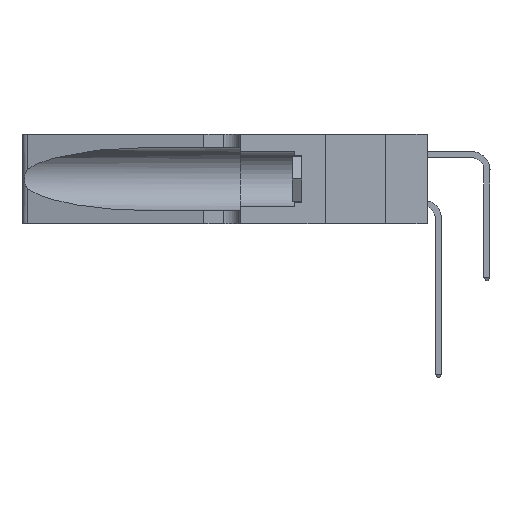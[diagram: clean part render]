
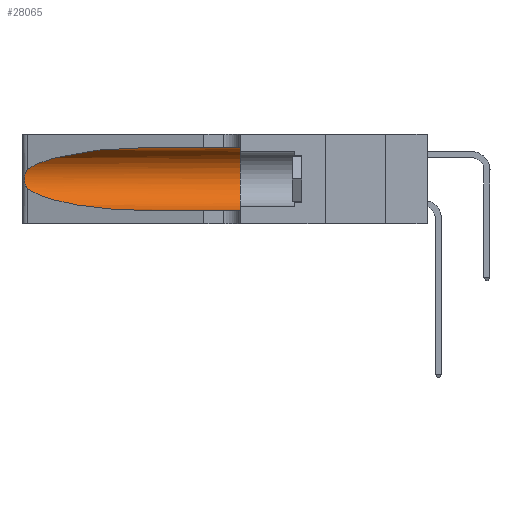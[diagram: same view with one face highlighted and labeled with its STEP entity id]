
A CAD part, left-side view. The second image highlights one B-rep face of the part: STEP entity #28065.
In plain terms, the highlighted cylindrical face has radius 3.308 mm (diameter 6.617 mm), a partial arc.
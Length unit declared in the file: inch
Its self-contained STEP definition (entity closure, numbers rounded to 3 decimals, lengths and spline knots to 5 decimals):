
#1088 = VERTEX_POINT ( 'NONE', #12390 ) ;
#1536 = AXIS2_PLACEMENT_3D ( 'NONE', #12603, #27786, #14799 ) ;
#1620 = CARTESIAN_POINT ( 'NONE',  ( 0.25856, 1.23593, 0.16098 ) ) ;
#2555 = EDGE_CURVE ( 'NONE', #1088, #3477, #3998, .T. ) ;
#2983 = DIRECTION ( 'NONE',  ( 0., -1., 0. ) ) ;
#3477 = VERTEX_POINT ( 'NONE', #13409 ) ;
#3913 = CARTESIAN_POINT ( 'NONE',  ( 0.25487, 1.22718, 0.14631 ) ) ;
#3923 = CARTESIAN_POINT ( 'NONE',  ( 0.25639, 1.23186, 0.15144 ) ) ;
#3998 = B_SPLINE_CURVE_WITH_KNOTS ( 'NONE', 3,
 ( #19181, #21332, #8282, #23526, #10497, #25715, #12701, #27890, #14899, #1620, #17091, #3923, #19275, #6166 ),
 .UNSPECIFIED., .F., .F.,
 ( 4, 2, 2, 2, 2, 2, 4 ),
 ( 0., 0.00027, 0.00053, 0.00107, 0.0016, 0.00187, 0.00214 ),
 .UNSPECIFIED. ) ;
#5432 = VECTOR ( 'NONE', #28395, 39.37008 ) ;
#5840 = CARTESIAN_POINT ( 'NONE',  ( 0.1305, 0.35, 0.31525 ) ) ;
#6016 = VERTEX_POINT ( 'NONE', #20432 ) ;
#6166 = CARTESIAN_POINT ( 'NONE',  ( 0.25487, 1.22718, 0.14631 ) ) ;
#6341 = FACE_OUTER_BOUND ( 'NONE', #9222, .T. ) ;
#6517 = DIRECTION ( 'NONE',  ( 0., 0., -1. ) ) ;
#6996 = DIRECTION ( 'NONE',  ( 0., -1., 0. ) ) ;
#8065 = CIRCLE ( 'NONE', #1536, 0.13025 ) ;
#8282 = CARTESIAN_POINT ( 'NONE',  ( 0.25639, 1.23184, 0.21858 ) ) ;
#8372 = CARTESIAN_POINT ( 'NONE',  ( 0.1305, 0.72297, 0.05475 ) ) ;
#9222 = EDGE_LOOP ( 'NONE', ( #16063, #11621, #13001, #24546, #14367, #15057 ) ) ;
#9246 = VERTEX_POINT ( 'NONE', #5840 ) ;
#9390 = VERTEX_POINT ( 'NONE', #28125 ) ;
#9672 =( BOUNDED_CURVE ( )  B_SPLINE_CURVE ( 3, ( #18338, #26934, #24857, #11829 ),
 .UNSPECIFIED., .F., .T. ) 
 B_SPLINE_CURVE_WITH_KNOTS ( ( 4, 4 ),
 ( 1.5708, 2.84003 ),
 .UNSPECIFIED. ) 
 CURVE ( )  GEOMETRIC_REPRESENTATION_ITEM ( )  RATIONAL_B_SPLINE_CURVE ( ( 1., 0.87, 0.87, 1. ) ) 
 REPRESENTATION_ITEM ( '' )  );
#10497 = CARTESIAN_POINT ( 'NONE',  ( 0.25854, 1.2359, 0.20912 ) ) ;
#11621 = ORIENTED_EDGE ( 'NONE', *, *, #2555, .T. ) ;
#11829 = CARTESIAN_POINT ( 'NONE',  ( 0.25487, 1.22718, 0.22369 ) ) ;
#12390 = CARTESIAN_POINT ( 'NONE',  ( 0.25487, 1.22718, 0.22369 ) ) ;
#12603 = CARTESIAN_POINT ( 'NONE',  ( 0.1305, 0.35, 0.185 ) ) ;
#12701 = CARTESIAN_POINT ( 'NONE',  ( 0.26075, 1.23896, 0.19203 ) ) ;
#13001 = ORIENTED_EDGE ( 'NONE', *, *, #20253, .T. ) ;
#13203 = CARTESIAN_POINT ( 'NONE',  ( 0.1305, 1.61858, 0.05475 ) ) ;
#13409 = CARTESIAN_POINT ( 'NONE',  ( 0.25487, 1.22718, 0.14631 ) ) ;
#14367 = ORIENTED_EDGE ( 'NONE', *, *, #20207, .F. ) ;
#14752 =( BOUNDED_CURVE ( )  B_SPLINE_CURVE ( 3, ( #3913, #17085, #21414, #8372 ),
 .UNSPECIFIED., .F., .T. ) 
 B_SPLINE_CURVE_WITH_KNOTS ( ( 4, 4 ),
 ( 3.44316, 4.71239 ),
 .UNSPECIFIED. ) 
 CURVE ( )  GEOMETRIC_REPRESENTATION_ITEM ( )  RATIONAL_B_SPLINE_CURVE ( ( 1., 0.87, 0.87, 1. ) ) 
 REPRESENTATION_ITEM ( '' )  );
#14799 = DIRECTION ( 'NONE',  ( 0., 0., 1. ) ) ;
#14899 = CARTESIAN_POINT ( 'NONE',  ( 0.26017, 1.23833, 0.17102 ) ) ;
#15057 = ORIENTED_EDGE ( 'NONE', *, *, #26070, .F. ) ;
#16063 = ORIENTED_EDGE ( 'NONE', *, *, #21930, .T. ) ;
#17021 = VECTOR ( 'NONE', #2983, 39.37008 ) ;
#17085 = CARTESIAN_POINT ( 'NONE',  ( 0.2373, 1.15595, 0.08982 ) ) ;
#17091 = CARTESIAN_POINT ( 'NONE',  ( 0.25789, 1.23486, 0.15765 ) ) ;
#18338 = CARTESIAN_POINT ( 'NONE',  ( 0.1305, 0.72297, 0.31525 ) ) ;
#18398 = CARTESIAN_POINT ( 'NONE',  ( 0.1305, 1.61858, 0.31525 ) ) ;
#19181 = CARTESIAN_POINT ( 'NONE',  ( 0.25487, 1.22718, 0.22369 ) ) ;
#19275 = CARTESIAN_POINT ( 'NONE',  ( 0.25555, 1.22993, 0.14849 ) ) ;
#20082 = CARTESIAN_POINT ( 'NONE',  ( 0.1305, 1.61858, 0.185 ) ) ;
#20207 = EDGE_CURVE ( 'NONE', #9246, #6016, #8065, .T. ) ;
#20253 = EDGE_CURVE ( 'NONE', #3477, #9390, #14752, .T. ) ;
#20432 = CARTESIAN_POINT ( 'NONE',  ( 0.1305, 0.35, 0.05475 ) ) ;
#20837 = AXIS2_PLACEMENT_3D ( 'NONE', #20082, #6996, #6517 ) ;
#21332 = CARTESIAN_POINT ( 'NONE',  ( 0.25555, 1.22994, 0.2215 ) ) ;
#21414 = CARTESIAN_POINT ( 'NONE',  ( 0.18966, 0.96281, 0.05475 ) ) ;
#21930 = EDGE_CURVE ( 'NONE', #27591, #1088, #9672, .T. ) ;
#22356 = CYLINDRICAL_SURFACE ( 'NONE', #20837, 0.13025 ) ;
#22808 = LINE ( 'NONE', #13203, #5432 ) ;
#23526 = CARTESIAN_POINT ( 'NONE',  ( 0.25787, 1.23484, 0.2124 ) ) ;
#24546 = ORIENTED_EDGE ( 'NONE', *, *, #25156, .T. ) ;
#24857 = CARTESIAN_POINT ( 'NONE',  ( 0.2373, 1.15595, 0.28018 ) ) ;
#25156 = EDGE_CURVE ( 'NONE', #9390, #6016, #22808, .T. ) ;
#25715 = CARTESIAN_POINT ( 'NONE',  ( 0.26018, 1.23835, 0.19895 ) ) ;
#26070 = EDGE_CURVE ( 'NONE', #27591, #9246, #27865, .T. ) ;
#26934 = CARTESIAN_POINT ( 'NONE',  ( 0.18966, 0.96281, 0.31525 ) ) ;
#27591 = VERTEX_POINT ( 'NONE', #28076 ) ;
#27786 = DIRECTION ( 'NONE',  ( 0., 1., 0. ) ) ;
#27865 = LINE ( 'NONE', #18398, #17021 ) ;
#27890 = CARTESIAN_POINT ( 'NONE',  ( 0.26075, 1.23896, 0.178 ) ) ;
#28065 = ADVANCED_FACE ( 'NONE', ( #6341 ), #22356, .F. ) ;
#28076 = CARTESIAN_POINT ( 'NONE',  ( 0.1305, 0.72297, 0.31525 ) ) ;
#28125 = CARTESIAN_POINT ( 'NONE',  ( 0.1305, 0.72297, 0.05475 ) ) ;
#28395 = DIRECTION ( 'NONE',  ( 0., -1., 0. ) ) ;
